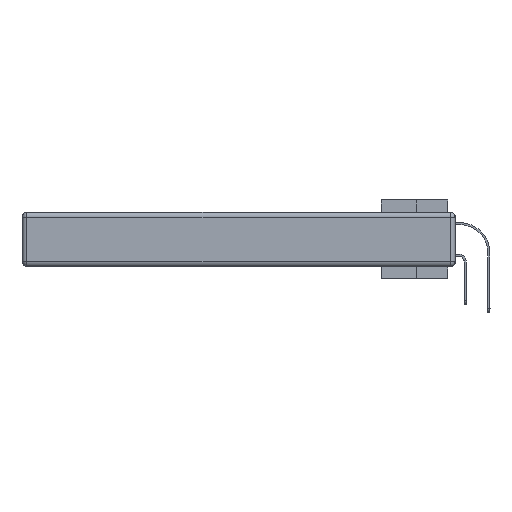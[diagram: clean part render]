
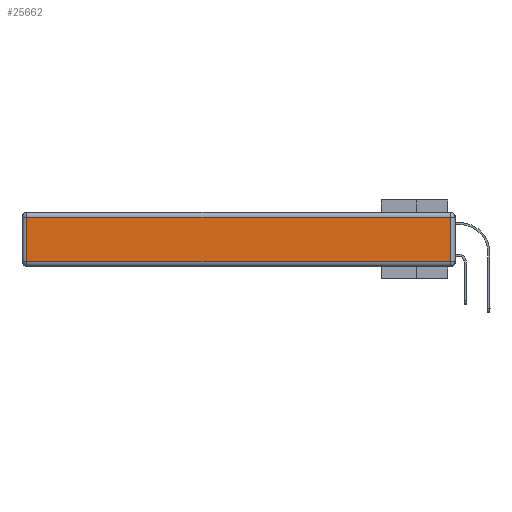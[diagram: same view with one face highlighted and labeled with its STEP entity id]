
A CAD part, left-side view. The second image highlights one B-rep face of the part: STEP entity #25662.
In plain terms, the highlighted planar face has unit normal (-1, 0, 0).
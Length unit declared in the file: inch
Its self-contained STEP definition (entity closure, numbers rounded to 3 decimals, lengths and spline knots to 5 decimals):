
#152 = LINE ( 'NONE', #33766, #40635 ) ;
#494 = DIRECTION ( 'NONE',  ( -1., 0., 0. ) ) ;
#3045 = CARTESIAN_POINT ( 'NONE',  ( 0., 0., -0.313 ) ) ;
#3161 = DIRECTION ( 'NONE',  ( 0., 1., 0. ) ) ;
#6482 = DIRECTION ( 'NONE',  ( 0., 0., 1. ) ) ;
#8945 = VERTEX_POINT ( 'NONE', #18659 ) ;
#8992 = CARTESIAN_POINT ( 'NONE',  ( 0., 2.72, -0.313 ) ) ;
#9635 = ORIENTED_EDGE ( 'NONE', *, *, #27373, .T. ) ;
#10752 = ORIENTED_EDGE ( 'NONE', *, *, #20894, .T. ) ;
#10965 = DIRECTION ( 'NONE',  ( 0., 0., 1. ) ) ;
#11102 = ORIENTED_EDGE ( 'NONE', *, *, #16077, .T. ) ;
#13130 = ORIENTED_EDGE ( 'NONE', *, *, #13912, .T. ) ;
#13912 = EDGE_CURVE ( 'NONE', #33098, #39635, #23089, .T. ) ;
#16077 = EDGE_CURVE ( 'NONE', #8945, #33098, #33058, .T. ) ;
#16669 = VERTEX_POINT ( 'NONE', #37311 ) ;
#17497 = PLANE ( 'NONE',  #38059 ) ;
#18399 = VECTOR ( 'NONE', #42570, 39.37008 ) ;
#18659 = CARTESIAN_POINT ( 'NONE',  ( 0., 0.03, -0.03 ) ) ;
#20894 = EDGE_CURVE ( 'NONE', #16669, #8945, #152, .T. ) ;
#23089 = LINE ( 'NONE', #42977, #33864 ) ;
#23109 = LINE ( 'NONE', #3045, #18399 ) ;
#24837 = VECTOR ( 'NONE', #3161, 39.37008 ) ;
#25662 = ADVANCED_FACE ( 'NONE', ( #40636 ), #17497, .T. ) ;
#27373 = EDGE_CURVE ( 'NONE', #39635, #16669, #23109, .T. ) ;
#28015 = CARTESIAN_POINT ( 'NONE',  ( 0., 2.72, -0.03 ) ) ;
#29777 = CARTESIAN_POINT ( 'NONE',  ( 0., 2.75, -0.03 ) ) ;
#32918 = DIRECTION ( 'NONE',  ( 0., 0., -1. ) ) ;
#33058 = LINE ( 'NONE', #29777, #24837 ) ;
#33098 = VERTEX_POINT ( 'NONE', #28015 ) ;
#33766 = CARTESIAN_POINT ( 'NONE',  ( 0., 0.03, -0.343 ) ) ;
#33864 = VECTOR ( 'NONE', #32918, 39.37008 ) ;
#37311 = CARTESIAN_POINT ( 'NONE',  ( 0., 0.03, -0.313 ) ) ;
#38059 = AXIS2_PLACEMENT_3D ( 'NONE', #40864, #494, #10965 ) ;
#39635 = VERTEX_POINT ( 'NONE', #8992 ) ;
#39766 = EDGE_LOOP ( 'NONE', ( #9635, #10752, #11102, #13130 ) ) ;
#40635 = VECTOR ( 'NONE', #6482, 39.37008 ) ;
#40636 = FACE_OUTER_BOUND ( 'NONE', #39766, .T. ) ;
#40864 = CARTESIAN_POINT ( 'NONE',  ( 0., 0., -0.343 ) ) ;
#42570 = DIRECTION ( 'NONE',  ( 0., -1., 0. ) ) ;
#42977 = CARTESIAN_POINT ( 'NONE',  ( 0., 2.72, -0.343 ) ) ;
